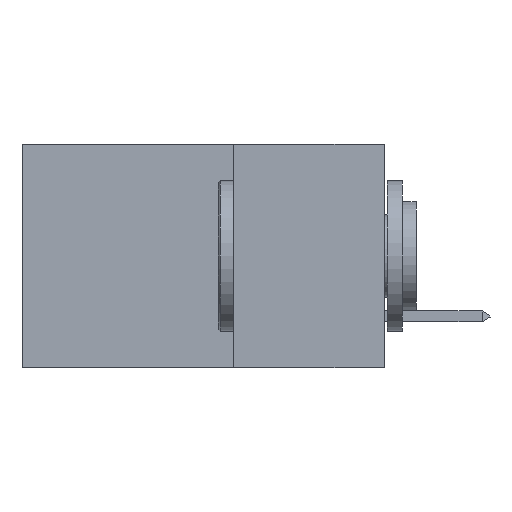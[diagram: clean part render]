
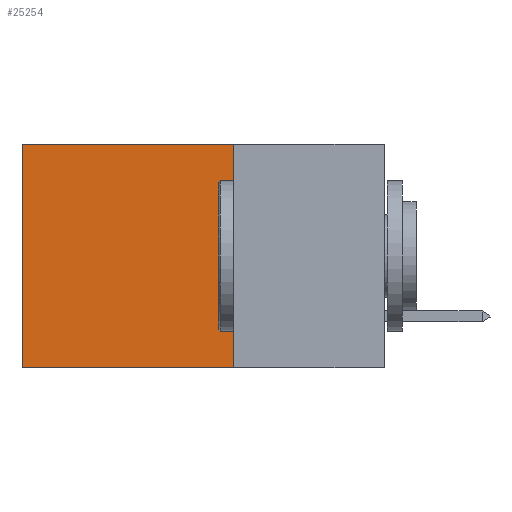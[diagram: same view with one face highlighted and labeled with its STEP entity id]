
A CAD part, left-side view. The second image highlights one B-rep face of the part: STEP entity #25254.
In plain terms, the highlighted planar face has unit normal (-1, 0, 0).
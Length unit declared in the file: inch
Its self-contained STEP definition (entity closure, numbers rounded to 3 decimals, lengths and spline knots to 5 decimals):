
#3721 = CARTESIAN_POINT ( 'NONE',  ( 0.2875, 0.25, 0. ) ) ;
#4454 = VERTEX_POINT ( 'NONE', #41121 ) ;
#5135 = EDGE_LOOP ( 'NONE', ( #39461, #32277, #8379, #8786 ) ) ;
#5175 = VERTEX_POINT ( 'NONE', #36969 ) ;
#5691 = DIRECTION ( 'NONE',  ( 0., 0., -1. ) ) ;
#8379 = ORIENTED_EDGE ( 'NONE', *, *, #30460, .F. ) ;
#8565 = DIRECTION ( 'NONE',  ( 0., 0., -1. ) ) ;
#8786 = ORIENTED_EDGE ( 'NONE', *, *, #33662, .T. ) ;
#9611 = PLANE ( 'NONE',  #34446 ) ;
#9644 = DIRECTION ( 'NONE',  ( 0., 0., -1. ) ) ;
#12810 = CARTESIAN_POINT ( 'NONE',  ( 0.2875, 0.25, 0. ) ) ;
#17242 = VECTOR ( 'NONE', #8565, 39.37008 ) ;
#17781 = EDGE_CURVE ( 'NONE', #36568, #24482, #27891, .T. ) ;
#18603 = EDGE_CURVE ( 'NONE', #4454, #24482, #40113, .T. ) ;
#18723 = CARTESIAN_POINT ( 'NONE',  ( 0.2875, 0.6, 0. ) ) ;
#18931 = VECTOR ( 'NONE', #36021, 39.37008 ) ;
#19701 = VECTOR ( 'NONE', #9644, 39.37008 ) ;
#20003 = CARTESIAN_POINT ( 'NONE',  ( 0.2875, 0.25, 0. ) ) ;
#23406 = LINE ( 'NONE', #3721, #18931 ) ;
#24482 = VERTEX_POINT ( 'NONE', #30315 ) ;
#24518 = DIRECTION ( 'NONE',  ( 0., 1., 0. ) ) ;
#25254 = ADVANCED_FACE ( 'NONE', ( #33370 ), #9611, .F. ) ;
#27891 = LINE ( 'NONE', #44692, #17242 ) ;
#27978 = CARTESIAN_POINT ( 'NONE',  ( 0.2875, 0.25, -0.37 ) ) ;
#30315 = CARTESIAN_POINT ( 'NONE',  ( 0.2875, 0.6, -0.37 ) ) ;
#30460 = EDGE_CURVE ( 'NONE', #5175, #4454, #42135, .T. ) ;
#30789 = DIRECTION ( 'NONE',  ( 1., 0., 0. ) ) ;
#32277 = ORIENTED_EDGE ( 'NONE', *, *, #18603, .F. ) ;
#33370 = FACE_OUTER_BOUND ( 'NONE', #5135, .T. ) ;
#33662 = EDGE_CURVE ( 'NONE', #5175, #36568, #23406, .T. ) ;
#33930 = VECTOR ( 'NONE', #24518, 39.37008 ) ;
#34446 = AXIS2_PLACEMENT_3D ( 'NONE', #20003, #30789, #5691 ) ;
#36021 = DIRECTION ( 'NONE',  ( 0., 1., 0. ) ) ;
#36568 = VERTEX_POINT ( 'NONE', #18723 ) ;
#36969 = CARTESIAN_POINT ( 'NONE',  ( 0.2875, 0.25, 0. ) ) ;
#39461 = ORIENTED_EDGE ( 'NONE', *, *, #17781, .T. ) ;
#40113 = LINE ( 'NONE', #27978, #33930 ) ;
#41121 = CARTESIAN_POINT ( 'NONE',  ( 0.2875, 0.25, -0.37 ) ) ;
#42135 = LINE ( 'NONE', #12810, #19701 ) ;
#44692 = CARTESIAN_POINT ( 'NONE',  ( 0.2875, 0.6, 0. ) ) ;
